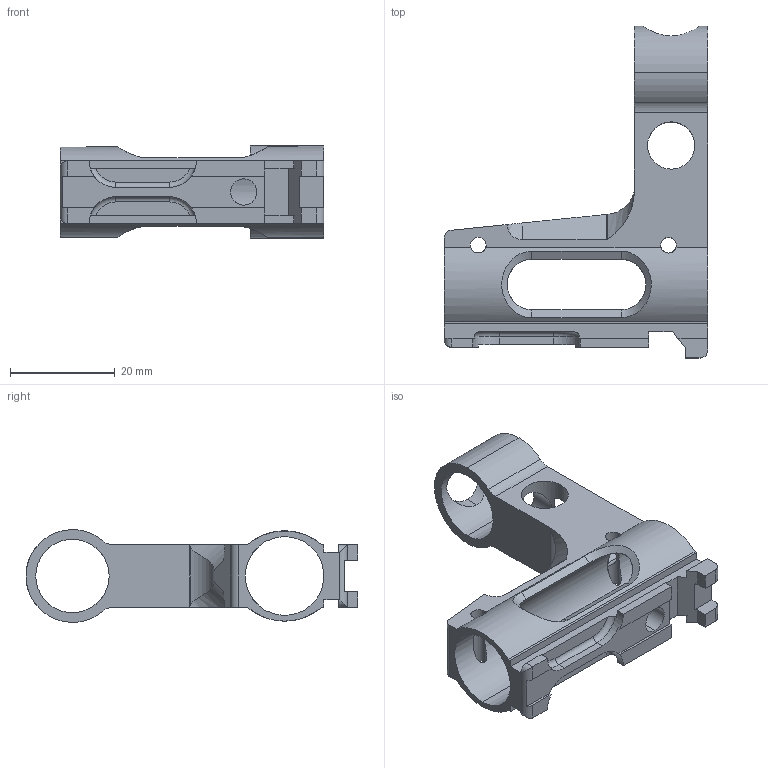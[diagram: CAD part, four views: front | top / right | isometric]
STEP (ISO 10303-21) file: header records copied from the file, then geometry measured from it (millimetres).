
FILE_DESCRIPTION (( 'STEP AP214' ), '1' );
FILE_NAME ('Front_Sight.STEP', '2013-06-19T08:07:47', ( 'fireraisr' ), ( '' ), 'SwSTEP 2.0', 'SolidWorks 2012', '' );
FILE_SCHEMA (( 'AUTOMOTIVE_DESIGN' ));
Length unit declared in the file: millimetre
Products named in the file (1): Front_Sight
Bounding box: 50.3 x 63.3 x 17.7 mm (x, y, z)
Volume: 8990.3 mm3; surface area: 8263.6 mm2
Topology: 1 solids, 1 shells, 129 faces, 390 edges, 254 vertices
Faces by surface type: plane 57, cylinder 54, bspline 10, torus 8
Entity records: 5807 total; most frequent: CARTESIAN_POINT 2343, ORIENTED_EDGE 780, DIRECTION 644, EDGE_CURVE 390, VERTEX_POINT 254, AXIS2_PLACEMENT_3D 218, LINE 208, VECTOR 208
